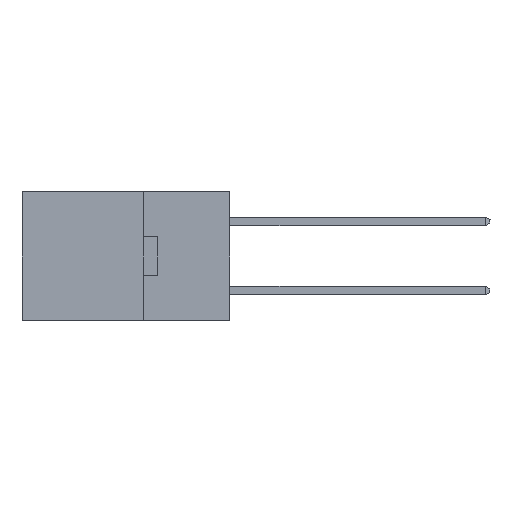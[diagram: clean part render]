
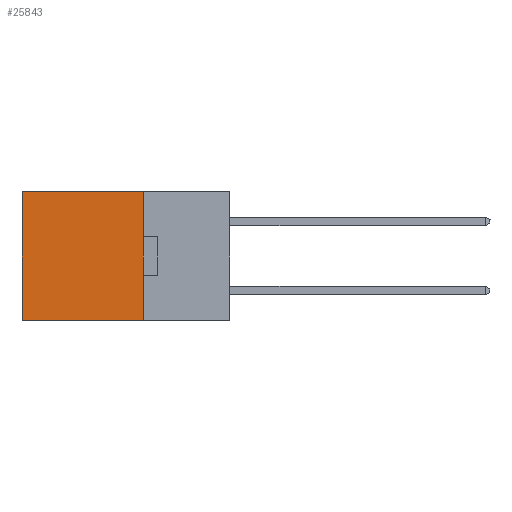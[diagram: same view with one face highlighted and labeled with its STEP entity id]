
A CAD part, left-side view. The second image highlights one B-rep face of the part: STEP entity #25843.
In plain terms, the highlighted planar face has unit normal (-1, 0, 0).
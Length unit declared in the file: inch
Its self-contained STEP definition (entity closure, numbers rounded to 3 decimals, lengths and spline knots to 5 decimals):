
#132 = EDGE_CURVE ( 'NONE', #19149, #19515, #18994, .T. ) ;
#1499 = VERTEX_POINT ( 'NONE', #4656 ) ;
#1614 = DIRECTION ( 'NONE',  ( 0., 0., -1. ) ) ;
#1821 = FACE_OUTER_BOUND ( 'NONE', #23511, .T. ) ;
#2038 = ORIENTED_EDGE ( 'NONE', *, *, #132, .F. ) ;
#2739 = EDGE_CURVE ( 'NONE', #13027, #1499, #4204, .T. ) ;
#2865 = VECTOR ( 'NONE', #17138, 39.37008 ) ;
#4204 = LINE ( 'NONE', #14771, #12541 ) ;
#4281 = DIRECTION ( 'NONE',  ( 1., 0., 0. ) ) ;
#4656 = CARTESIAN_POINT ( 'NONE',  ( 0.2615, 0.6, -0.37 ) ) ;
#5221 = VECTOR ( 'NONE', #24568, 39.37008 ) ;
#5336 = CARTESIAN_POINT ( 'NONE',  ( 0.2615, 0.25, 0. ) ) ;
#5413 = ORIENTED_EDGE ( 'NONE', *, *, #2739, .T. ) ;
#8774 = CARTESIAN_POINT ( 'NONE',  ( 0.2615, 0.25, -0.37 ) ) ;
#10554 = VECTOR ( 'NONE', #1614, 39.37008 ) ;
#12541 = VECTOR ( 'NONE', #12897, 39.37008 ) ;
#12897 = DIRECTION ( 'NONE',  ( 0., 0., -1. ) ) ;
#13027 = VERTEX_POINT ( 'NONE', #16213 ) ;
#13124 = DIRECTION ( 'NONE',  ( 0., 0., -1. ) ) ;
#13273 = PLANE ( 'NONE',  #17491 ) ;
#14771 = CARTESIAN_POINT ( 'NONE',  ( 0.2615, 0.6, -0.37 ) ) ;
#15467 = LINE ( 'NONE', #26742, #5221 ) ;
#16213 = CARTESIAN_POINT ( 'NONE',  ( 0.2615, 0.6, 0. ) ) ;
#16533 = ORIENTED_EDGE ( 'NONE', *, *, #27277, .T. ) ;
#16615 = ORIENTED_EDGE ( 'NONE', *, *, #26204, .F. ) ;
#16856 = LINE ( 'NONE', #23068, #2865 ) ;
#17138 = DIRECTION ( 'NONE',  ( 0., 1., 0. ) ) ;
#17491 = AXIS2_PLACEMENT_3D ( 'NONE', #8774, #4281, #13124 ) ;
#18994 = LINE ( 'NONE', #21596, #10554 ) ;
#19149 = VERTEX_POINT ( 'NONE', #5336 ) ;
#19515 = VERTEX_POINT ( 'NONE', #24955 ) ;
#21596 = CARTESIAN_POINT ( 'NONE',  ( 0.2615, 0.25, -0.37 ) ) ;
#23068 = CARTESIAN_POINT ( 'NONE',  ( 0.2615, 0.25, -0.37 ) ) ;
#23511 = EDGE_LOOP ( 'NONE', ( #5413, #16615, #2038, #16533 ) ) ;
#24568 = DIRECTION ( 'NONE',  ( 0., 1., 0. ) ) ;
#24955 = CARTESIAN_POINT ( 'NONE',  ( 0.2615, 0.25, -0.37 ) ) ;
#25843 = ADVANCED_FACE ( 'NONE', ( #1821 ), #13273, .F. ) ;
#26204 = EDGE_CURVE ( 'NONE', #19515, #1499, #16856, .T. ) ;
#26742 = CARTESIAN_POINT ( 'NONE',  ( 0.2615, 0.25, 0. ) ) ;
#27277 = EDGE_CURVE ( 'NONE', #19149, #13027, #15467, .T. ) ;
